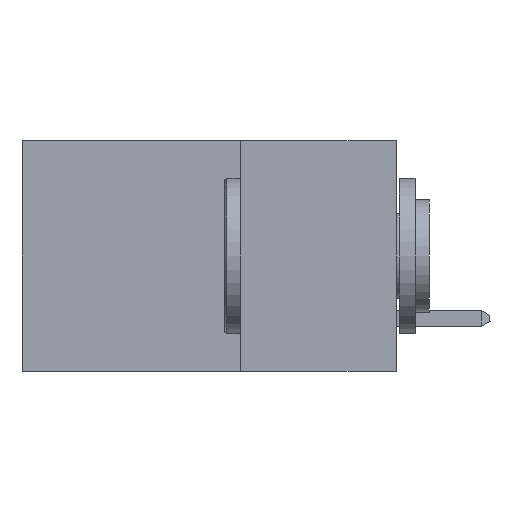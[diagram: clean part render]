
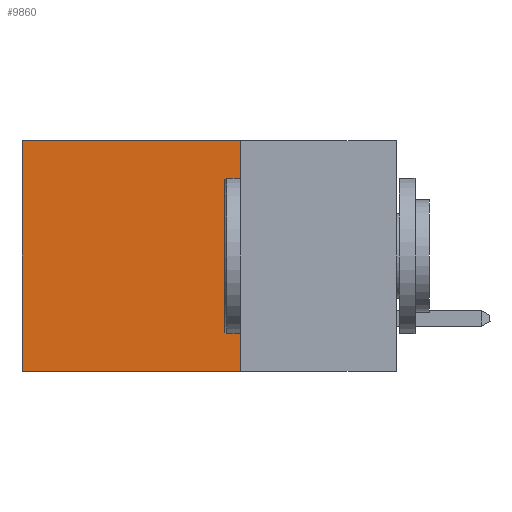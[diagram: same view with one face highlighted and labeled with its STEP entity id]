
A CAD part, left-side view. The second image highlights one B-rep face of the part: STEP entity #9860.
In plain terms, the highlighted planar face has unit normal (-1, 0, 0).
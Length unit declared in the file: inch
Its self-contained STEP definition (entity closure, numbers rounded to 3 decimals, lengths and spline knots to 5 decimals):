
#760 = FACE_OUTER_BOUND ( 'NONE', #6705, .T. ) ;
#1073 = VECTOR ( 'NONE', #5221, 39.37008 ) ;
#1549 = EDGE_CURVE ( 'NONE', #4051, #6306, #6761, .T. ) ;
#1593 = LINE ( 'NONE', #8355, #7273 ) ;
#2086 = CARTESIAN_POINT ( 'NONE',  ( 0.298, 0.25, 0. ) ) ;
#2140 = EDGE_CURVE ( 'NONE', #12528, #13202, #7285, .T. ) ;
#2488 = CARTESIAN_POINT ( 'NONE',  ( 0.298, 0.25, -0.37 ) ) ;
#2770 = DIRECTION ( 'NONE',  ( 0., 0., -1. ) ) ;
#2784 = CARTESIAN_POINT ( 'NONE',  ( 0.298, 0.6, 0. ) ) ;
#3676 = ORIENTED_EDGE ( 'NONE', *, *, #1549, .T. ) ;
#4051 = VERTEX_POINT ( 'NONE', #9696 ) ;
#4059 = LINE ( 'NONE', #10815, #1073 ) ;
#4220 = VECTOR ( 'NONE', #13236, 39.37008 ) ;
#5221 = DIRECTION ( 'NONE',  ( 0., 0., -1. ) ) ;
#5494 = CARTESIAN_POINT ( 'NONE',  ( 0.298, 0.25, -0.37 ) ) ;
#6209 = CARTESIAN_POINT ( 'NONE',  ( 0.298, 0.6, -0.37 ) ) ;
#6306 = VERTEX_POINT ( 'NONE', #2784 ) ;
#6705 = EDGE_LOOP ( 'NONE', ( #11425, #12255, #13610, #3676 ) ) ;
#6761 = LINE ( 'NONE', #2086, #7120 ) ;
#6769 = AXIS2_PLACEMENT_3D ( 'NONE', #8428, #9532, #2770 ) ;
#7120 = VECTOR ( 'NONE', #7350, 39.37008 ) ;
#7273 = VECTOR ( 'NONE', #9467, 39.37008 ) ;
#7285 = LINE ( 'NONE', #5494, #4220 ) ;
#7350 = DIRECTION ( 'NONE',  ( 0., 1., 0. ) ) ;
#7471 = EDGE_CURVE ( 'NONE', #4051, #12528, #1593, .T. ) ;
#8355 = CARTESIAN_POINT ( 'NONE',  ( 0.298, 0.25, 0. ) ) ;
#8428 = CARTESIAN_POINT ( 'NONE',  ( 0.298, 0.25, 0. ) ) ;
#9467 = DIRECTION ( 'NONE',  ( 0., 0., -1. ) ) ;
#9532 = DIRECTION ( 'NONE',  ( 1., 0., 0. ) ) ;
#9696 = CARTESIAN_POINT ( 'NONE',  ( 0.298, 0.25, 0. ) ) ;
#9860 = ADVANCED_FACE ( 'NONE', ( #760 ), #14105, .F. ) ;
#10815 = CARTESIAN_POINT ( 'NONE',  ( 0.298, 0.6, 0. ) ) ;
#11425 = ORIENTED_EDGE ( 'NONE', *, *, #11537, .T. ) ;
#11537 = EDGE_CURVE ( 'NONE', #6306, #13202, #4059, .T. ) ;
#12255 = ORIENTED_EDGE ( 'NONE', *, *, #2140, .F. ) ;
#12528 = VERTEX_POINT ( 'NONE', #2488 ) ;
#13202 = VERTEX_POINT ( 'NONE', #6209 ) ;
#13236 = DIRECTION ( 'NONE',  ( 0., 1., 0. ) ) ;
#13610 = ORIENTED_EDGE ( 'NONE', *, *, #7471, .F. ) ;
#14105 = PLANE ( 'NONE',  #6769 ) ;
